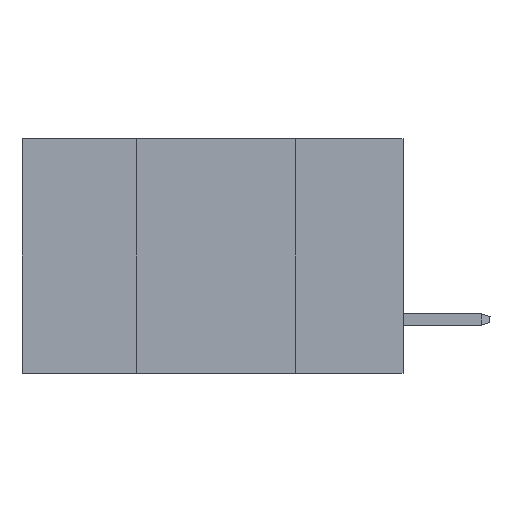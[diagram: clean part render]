
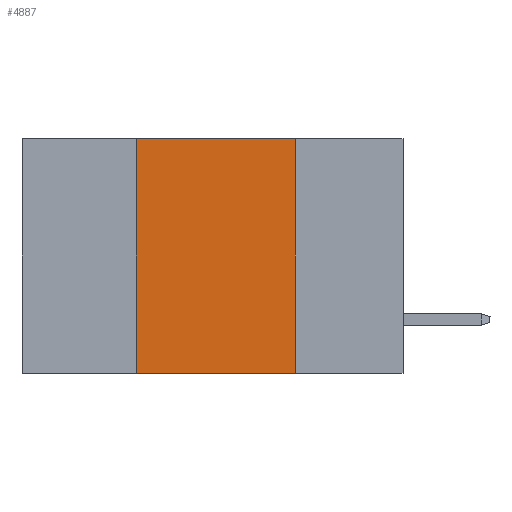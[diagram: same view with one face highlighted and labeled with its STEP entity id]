
A CAD part, left-side view. The second image highlights one B-rep face of the part: STEP entity #4887.
In plain terms, the highlighted planar face has unit normal (-1, 0, 0).
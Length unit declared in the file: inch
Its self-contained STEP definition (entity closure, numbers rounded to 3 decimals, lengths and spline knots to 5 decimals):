
#2175 = FACE_OUTER_BOUND ( 'NONE', #27727, .T. ) ;
#4887 = ADVANCED_FACE ( 'NONE', ( #2175 ), #13837, .F. ) ;
#6376 = VERTEX_POINT ( 'NONE', #18097 ) ;
#7076 = CARTESIAN_POINT ( 'NONE',  ( 0., 0.42, 0. ) ) ;
#10012 = CARTESIAN_POINT ( 'NONE',  ( 0., 0.6, 0. ) ) ;
#10395 = EDGE_CURVE ( 'NONE', #13677, #6376, #26417, .T. ) ;
#11199 = CARTESIAN_POINT ( 'NONE',  ( 0., 0.6, -0.37 ) ) ;
#11468 = VERTEX_POINT ( 'NONE', #48872 ) ;
#12893 = ORIENTED_EDGE ( 'NONE', *, *, #24114, .T. ) ;
#13222 = EDGE_CURVE ( 'NONE', #11468, #47341, #13635, .T. ) ;
#13635 = LINE ( 'NONE', #29187, #44950 ) ;
#13677 = VERTEX_POINT ( 'NONE', #17725 ) ;
#13837 = PLANE ( 'NONE',  #15738 ) ;
#14401 = CARTESIAN_POINT ( 'NONE',  ( 0., 0.6, 0. ) ) ;
#15738 = AXIS2_PLACEMENT_3D ( 'NONE', #10012, #18142, #45452 ) ;
#17725 = CARTESIAN_POINT ( 'NONE',  ( 0., 0.42, -0.37 ) ) ;
#18097 = CARTESIAN_POINT ( 'NONE',  ( 0., 0.42, 0. ) ) ;
#18142 = DIRECTION ( 'NONE',  ( 1., 0., 0. ) ) ;
#18235 = DIRECTION ( 'NONE',  ( 0., -1., 0. ) ) ;
#18845 = CARTESIAN_POINT ( 'NONE',  ( 0., 0.17, -0.37 ) ) ;
#22043 = LINE ( 'NONE', #14401, #27255 ) ;
#22898 = LINE ( 'NONE', #11199, #30852 ) ;
#24114 = EDGE_CURVE ( 'NONE', #13677, #47341, #22898, .T. ) ;
#26417 = LINE ( 'NONE', #7076, #34861 ) ;
#26740 = DIRECTION ( 'NONE',  ( 0., -1., 0. ) ) ;
#27218 = EDGE_CURVE ( 'NONE', #6376, #11468, #22043, .T. ) ;
#27255 = VECTOR ( 'NONE', #18235, 39.37008 ) ;
#27727 = EDGE_LOOP ( 'NONE', ( #43923, #30872, #28697, #12893 ) ) ;
#28697 = ORIENTED_EDGE ( 'NONE', *, *, #10395, .F. ) ;
#29187 = CARTESIAN_POINT ( 'NONE',  ( 0., 0.17, 0. ) ) ;
#30493 = DIRECTION ( 'NONE',  ( 0., 0., 1. ) ) ;
#30852 = VECTOR ( 'NONE', #26740, 39.37008 ) ;
#30872 = ORIENTED_EDGE ( 'NONE', *, *, #27218, .F. ) ;
#32744 = DIRECTION ( 'NONE',  ( 0., 0., -1. ) ) ;
#34861 = VECTOR ( 'NONE', #30493, 39.37008 ) ;
#43923 = ORIENTED_EDGE ( 'NONE', *, *, #13222, .F. ) ;
#44950 = VECTOR ( 'NONE', #32744, 39.37008 ) ;
#45452 = DIRECTION ( 'NONE',  ( 0., 0., -1. ) ) ;
#47341 = VERTEX_POINT ( 'NONE', #18845 ) ;
#48872 = CARTESIAN_POINT ( 'NONE',  ( 0., 0.17, 0. ) ) ;
